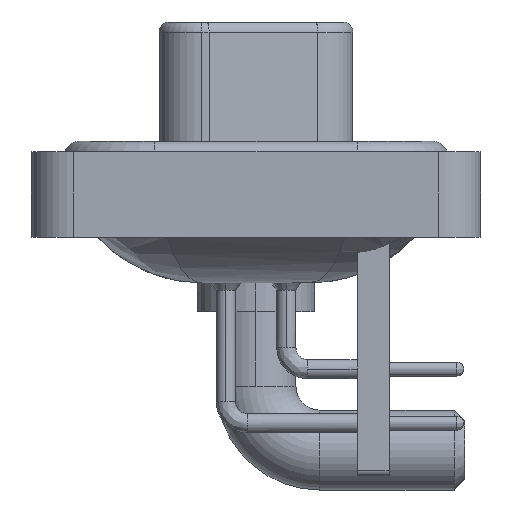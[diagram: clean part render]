
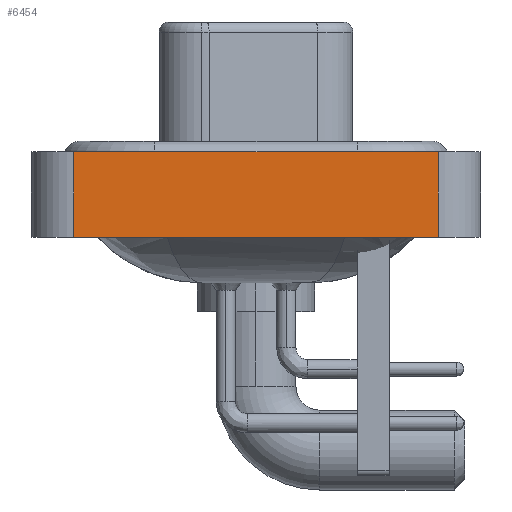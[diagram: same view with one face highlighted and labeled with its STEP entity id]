
A CAD part, left-side view. The second image highlights one B-rep face of the part: STEP entity #6454.
In plain terms, the highlighted planar face has unit normal (-1, 0, 0).
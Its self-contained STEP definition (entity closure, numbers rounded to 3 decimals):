
#62 = ORIENTED_EDGE ( 'NONE', *, *, #25045, .F. ) ;
#141 = VERTEX_POINT ( 'NONE', #24559 ) ;
#1599 = ORIENTED_EDGE ( 'NONE', *, *, #18460, .F. ) ;
#2028 = VERTEX_POINT ( 'NONE', #14087 ) ;
#2233 = EDGE_LOOP ( 'NONE', ( #4613, #62, #1599, #26495 ) ) ;
#2507 = AXIS2_PLACEMENT_3D ( 'NONE', #14515, #18662, #11771 ) ;
#3217 = LINE ( 'NONE', #19789, #7844 ) ;
#3784 = CARTESIAN_POINT ( 'NONE',  ( -7.35, 8.55, -3.6 ) ) ;
#4613 = ORIENTED_EDGE ( 'NONE', *, *, #20362, .T. ) ;
#6214 = LINE ( 'NONE', #15276, #12574 ) ;
#6454 = ADVANCED_FACE ( 'NONE', ( #19108 ), #16502, .T. ) ;
#7844 = VECTOR ( 'NONE', #22102, 1000. ) ;
#9318 = LINE ( 'NONE', #25580, #20475 ) ;
#11662 = DIRECTION ( 'NONE',  ( 0., 0., 1. ) ) ;
#11771 = DIRECTION ( 'NONE',  ( 0., 0., 1. ) ) ;
#12492 = VECTOR ( 'NONE', #11662, 1000. ) ;
#12574 = VECTOR ( 'NONE', #24325, 1000. ) ;
#14087 = CARTESIAN_POINT ( 'NONE',  ( -7.35, -8.55, 0.4 ) ) ;
#14515 = CARTESIAN_POINT ( 'NONE',  ( -7.35, -8.55, -3.6 ) ) ;
#15276 = CARTESIAN_POINT ( 'NONE',  ( -7.35, -8.55, -3.6 ) ) ;
#16245 = CARTESIAN_POINT ( 'NONE',  ( -7.35, 8.55, -3.6 ) ) ;
#16392 = LINE ( 'NONE', #16245, #12492 ) ;
#16502 = PLANE ( 'NONE',  #2507 ) ;
#17083 = VERTEX_POINT ( 'NONE', #3784 ) ;
#18460 = EDGE_CURVE ( 'NONE', #17083, #141, #16392, .T. ) ;
#18662 = DIRECTION ( 'NONE',  ( -1., 0., 0. ) ) ;
#19108 = FACE_OUTER_BOUND ( 'NONE', #2233, .T. ) ;
#19789 = CARTESIAN_POINT ( 'NONE',  ( -7.35, -8.55, 0.4 ) ) ;
#20362 = EDGE_CURVE ( 'NONE', #22247, #2028, #9318, .T. ) ;
#20475 = VECTOR ( 'NONE', #30327, 1000. ) ;
#22102 = DIRECTION ( 'NONE',  ( 0., -1., 0. ) ) ;
#22247 = VERTEX_POINT ( 'NONE', #29053 ) ;
#24325 = DIRECTION ( 'NONE',  ( 0., -1., 0. ) ) ;
#24559 = CARTESIAN_POINT ( 'NONE',  ( -7.35, 8.55, 0.4 ) ) ;
#25045 = EDGE_CURVE ( 'NONE', #141, #2028, #3217, .T. ) ;
#25580 = CARTESIAN_POINT ( 'NONE',  ( -7.35, -8.55, -3.6 ) ) ;
#26495 = ORIENTED_EDGE ( 'NONE', *, *, #28017, .T. ) ;
#28017 = EDGE_CURVE ( 'NONE', #17083, #22247, #6214, .T. ) ;
#29053 = CARTESIAN_POINT ( 'NONE',  ( -7.35, -8.55, -3.6 ) ) ;
#30327 = DIRECTION ( 'NONE',  ( 0., 0., 1. ) ) ;
